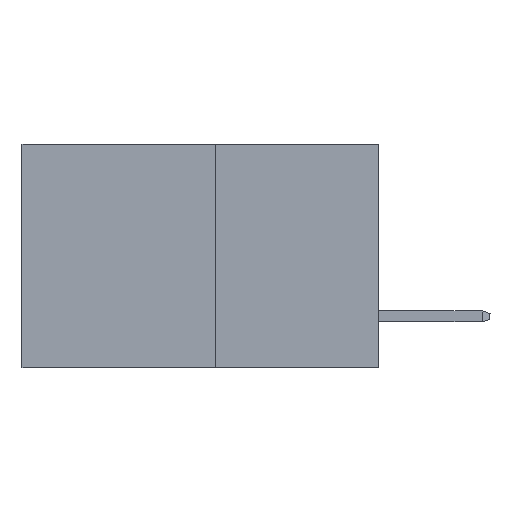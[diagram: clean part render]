
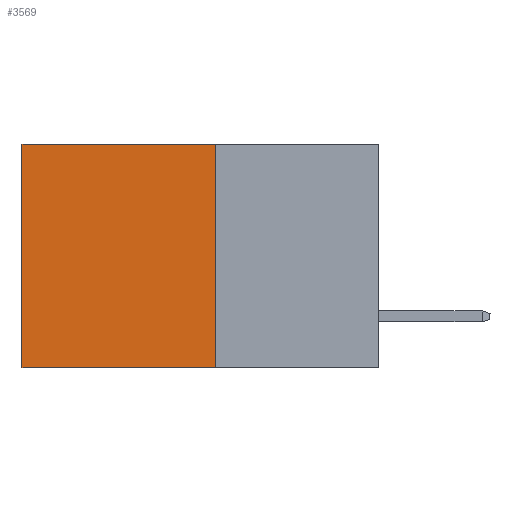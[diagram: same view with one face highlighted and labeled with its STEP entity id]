
A CAD part, left-side view. The second image highlights one B-rep face of the part: STEP entity #3569.
In plain terms, the highlighted planar face has unit normal (-1, 0, 0).
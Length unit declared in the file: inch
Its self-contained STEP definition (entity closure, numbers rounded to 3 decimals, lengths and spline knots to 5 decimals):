
#651 = VERTEX_POINT ( 'NONE', #22282 ) ;
#2215 = ORIENTED_EDGE ( 'NONE', *, *, #19458, .T. ) ;
#3381 = EDGE_CURVE ( 'NONE', #651, #12944, #25762, .T. ) ;
#3569 = ADVANCED_FACE ( 'NONE', ( #16123 ), #25866, .F. ) ;
#5043 = EDGE_CURVE ( 'NONE', #12944, #21236, #6166, .T. ) ;
#5709 = VECTOR ( 'NONE', #6877, 39.37008 ) ;
#5907 = ORIENTED_EDGE ( 'NONE', *, *, #5043, .F. ) ;
#6166 = LINE ( 'NONE', #22717, #15726 ) ;
#6713 = CARTESIAN_POINT ( 'NONE',  ( 0.277, 0.59, -0.37 ) ) ;
#6865 = AXIS2_PLACEMENT_3D ( 'NONE', #24639, #24158, #24031 ) ;
#6877 = DIRECTION ( 'NONE',  ( 0., 1., 0. ) ) ;
#7101 = CARTESIAN_POINT ( 'NONE',  ( 0.277, 0.27, -0.37 ) ) ;
#7125 = VECTOR ( 'NONE', #15241, 39.37008 ) ;
#7770 = LINE ( 'NONE', #25212, #7125 ) ;
#8338 = ORIENTED_EDGE ( 'NONE', *, *, #3381, .F. ) ;
#9278 = VERTEX_POINT ( 'NONE', #23400 ) ;
#12944 = VERTEX_POINT ( 'NONE', #7101 ) ;
#13043 = CARTESIAN_POINT ( 'NONE',  ( 0.277, 0.27, 0. ) ) ;
#13995 = EDGE_LOOP ( 'NONE', ( #18980, #5907, #8338, #2215 ) ) ;
#15241 = DIRECTION ( 'NONE',  ( 0., 0., -1. ) ) ;
#15726 = VECTOR ( 'NONE', #22660, 39.37008 ) ;
#16109 = EDGE_CURVE ( 'NONE', #9278, #21236, #7770, .T. ) ;
#16123 = FACE_OUTER_BOUND ( 'NONE', #13995, .T. ) ;
#18019 = DIRECTION ( 'NONE',  ( 0., 0., -1. ) ) ;
#18200 = CARTESIAN_POINT ( 'NONE',  ( 0.277, 0.27, -0.37 ) ) ;
#18980 = ORIENTED_EDGE ( 'NONE', *, *, #16109, .T. ) ;
#19458 = EDGE_CURVE ( 'NONE', #651, #9278, #21845, .T. ) ;
#20550 = VECTOR ( 'NONE', #18019, 39.37008 ) ;
#21236 = VERTEX_POINT ( 'NONE', #6713 ) ;
#21845 = LINE ( 'NONE', #13043, #5709 ) ;
#22282 = CARTESIAN_POINT ( 'NONE',  ( 0.277, 0.27, 0. ) ) ;
#22660 = DIRECTION ( 'NONE',  ( 0., 1., 0. ) ) ;
#22717 = CARTESIAN_POINT ( 'NONE',  ( 0.277, 0.27, -0.37 ) ) ;
#23400 = CARTESIAN_POINT ( 'NONE',  ( 0.277, 0.59, 0. ) ) ;
#24031 = DIRECTION ( 'NONE',  ( 0., 0., -1. ) ) ;
#24158 = DIRECTION ( 'NONE',  ( 1., 0., 0. ) ) ;
#24639 = CARTESIAN_POINT ( 'NONE',  ( 0.277, 0.27, -0.37 ) ) ;
#25212 = CARTESIAN_POINT ( 'NONE',  ( 0.277, 0.59, -0.37 ) ) ;
#25762 = LINE ( 'NONE', #18200, #20550 ) ;
#25866 = PLANE ( 'NONE',  #6865 ) ;
